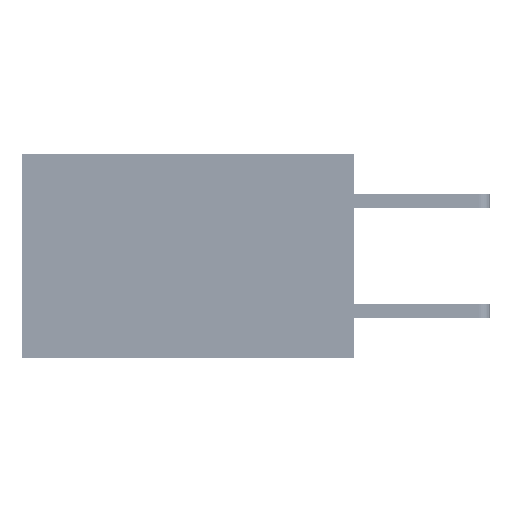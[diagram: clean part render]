
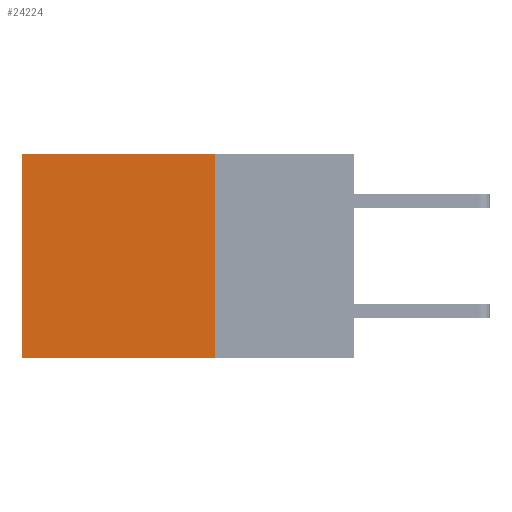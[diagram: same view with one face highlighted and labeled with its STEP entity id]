
A CAD part, left-side view. The second image highlights one B-rep face of the part: STEP entity #24224.
In plain terms, the highlighted planar face has unit normal (-1, 0, 0).
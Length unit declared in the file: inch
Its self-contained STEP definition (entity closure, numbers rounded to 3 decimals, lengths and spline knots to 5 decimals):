
#11 = CARTESIAN_POINT ( 'NONE',  ( 0.2875, 0.25, -0.37 ) ) ;
#3780 = CARTESIAN_POINT ( 'NONE',  ( 0.2875, 0.25, -0.37 ) ) ;
#4955 = ORIENTED_EDGE ( 'NONE', *, *, #9668, .F. ) ;
#5495 = DIRECTION ( 'NONE',  ( 0., 1., 0. ) ) ;
#6288 = VERTEX_POINT ( 'NONE', #35705 ) ;
#7191 = EDGE_LOOP ( 'NONE', ( #14718, #13721, #4955, #39446 ) ) ;
#8273 = EDGE_CURVE ( 'NONE', #6288, #11837, #40232, .T. ) ;
#8835 = VERTEX_POINT ( 'NONE', #13265 ) ;
#9668 = EDGE_CURVE ( 'NONE', #6288, #26231, #12274, .T. ) ;
#10163 = DIRECTION ( 'NONE',  ( 1., 0., 0. ) ) ;
#11837 = VERTEX_POINT ( 'NONE', #28037 ) ;
#12274 = LINE ( 'NONE', #31739, #25931 ) ;
#13265 = CARTESIAN_POINT ( 'NONE',  ( 0.2875, 0.6, -0.37 ) ) ;
#13721 = ORIENTED_EDGE ( 'NONE', *, *, #31094, .F. ) ;
#14718 = ORIENTED_EDGE ( 'NONE', *, *, #40429, .T. ) ;
#15470 = AXIS2_PLACEMENT_3D ( 'NONE', #17025, #10163, #35422 ) ;
#17025 = CARTESIAN_POINT ( 'NONE',  ( 0.2875, 0.25, 0. ) ) ;
#17273 = DIRECTION ( 'NONE',  ( 0., 1., 0. ) ) ;
#17890 = FACE_OUTER_BOUND ( 'NONE', #7191, .T. ) ;
#22288 = CARTESIAN_POINT ( 'NONE',  ( 0.2875, 0.6, 0. ) ) ;
#23003 = VECTOR ( 'NONE', #40091, 39.37008 ) ;
#24224 = ADVANCED_FACE ( 'NONE', ( #17890 ), #31029, .F. ) ;
#24327 = DIRECTION ( 'NONE',  ( 0., 0., -1. ) ) ;
#24793 = VECTOR ( 'NONE', #17273, 39.37008 ) ;
#25931 = VECTOR ( 'NONE', #24327, 39.37008 ) ;
#26231 = VERTEX_POINT ( 'NONE', #3780 ) ;
#28037 = CARTESIAN_POINT ( 'NONE',  ( 0.2875, 0.6, 0. ) ) ;
#31029 = PLANE ( 'NONE',  #15470 ) ;
#31094 = EDGE_CURVE ( 'NONE', #26231, #8835, #42778, .T. ) ;
#31739 = CARTESIAN_POINT ( 'NONE',  ( 0.2875, 0.25, 0. ) ) ;
#32222 = LINE ( 'NONE', #22288, #23003 ) ;
#32756 = CARTESIAN_POINT ( 'NONE',  ( 0.2875, 0.25, 0. ) ) ;
#33159 = VECTOR ( 'NONE', #5495, 39.37008 ) ;
#35422 = DIRECTION ( 'NONE',  ( 0., 0., -1. ) ) ;
#35705 = CARTESIAN_POINT ( 'NONE',  ( 0.2875, 0.25, 0. ) ) ;
#39446 = ORIENTED_EDGE ( 'NONE', *, *, #8273, .T. ) ;
#40091 = DIRECTION ( 'NONE',  ( 0., 0., -1. ) ) ;
#40232 = LINE ( 'NONE', #32756, #33159 ) ;
#40429 = EDGE_CURVE ( 'NONE', #11837, #8835, #32222, .T. ) ;
#42778 = LINE ( 'NONE', #11, #24793 ) ;
